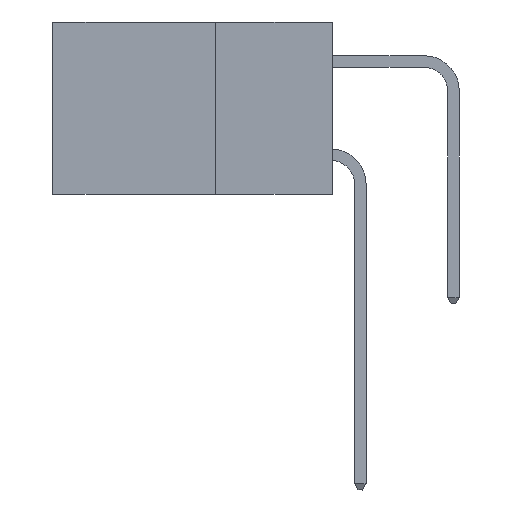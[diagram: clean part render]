
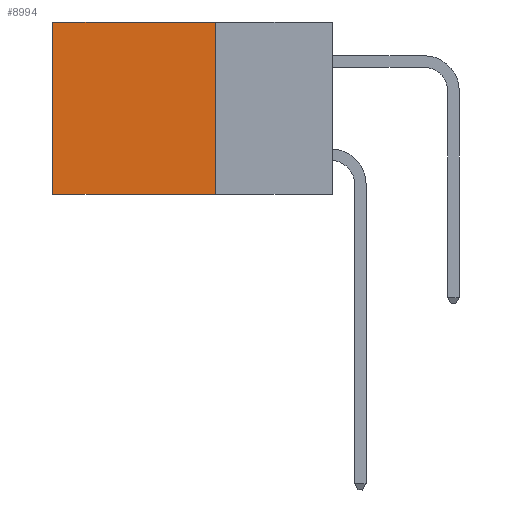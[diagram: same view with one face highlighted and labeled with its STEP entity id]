
A CAD part, left-side view. The second image highlights one B-rep face of the part: STEP entity #8994.
In plain terms, the highlighted planar face has unit normal (-1, 0, 0).
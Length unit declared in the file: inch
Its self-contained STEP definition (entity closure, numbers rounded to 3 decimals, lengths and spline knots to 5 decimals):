
#32 = PLANE ( 'NONE',  #10204 ) ;
#235 = LINE ( 'NONE', #8514, #19028 ) ;
#2487 = VECTOR ( 'NONE', #20587, 39.37008 ) ;
#2518 = LINE ( 'NONE', #22984, #2487 ) ;
#2733 = VERTEX_POINT ( 'NONE', #11501 ) ;
#2996 = CARTESIAN_POINT ( 'NONE',  ( 0.2615, 0.25, 0. ) ) ;
#5278 = EDGE_CURVE ( 'NONE', #16045, #2733, #235, .T. ) ;
#5744 = ORIENTED_EDGE ( 'NONE', *, *, #19781, .F. ) ;
#6216 = CARTESIAN_POINT ( 'NONE',  ( 0.2615, 0.25, -0.37 ) ) ;
#7022 = CARTESIAN_POINT ( 'NONE',  ( 0.2615, 0.25, 0. ) ) ;
#7184 = LINE ( 'NONE', #17378, #13124 ) ;
#7580 = DIRECTION ( 'NONE',  ( 0., 1., 0. ) ) ;
#8514 = CARTESIAN_POINT ( 'NONE',  ( 0.2615, 0.6, -0.37 ) ) ;
#8994 = ADVANCED_FACE ( 'NONE', ( #18244 ), #32, .F. ) ;
#9615 = VERTEX_POINT ( 'NONE', #6216 ) ;
#10204 = AXIS2_PLACEMENT_3D ( 'NONE', #24388, #17023, #25290 ) ;
#11501 = CARTESIAN_POINT ( 'NONE',  ( 0.2615, 0.6, -0.37 ) ) ;
#13116 = CARTESIAN_POINT ( 'NONE',  ( 0.2615, 0.6, 0. ) ) ;
#13124 = VECTOR ( 'NONE', #7580, 39.37008 ) ;
#13765 = EDGE_CURVE ( 'NONE', #16573, #16045, #14827, .T. ) ;
#14450 = ORIENTED_EDGE ( 'NONE', *, *, #13765, .T. ) ;
#14827 = LINE ( 'NONE', #7022, #17123 ) ;
#16045 = VERTEX_POINT ( 'NONE', #13116 ) ;
#16573 = VERTEX_POINT ( 'NONE', #2996 ) ;
#17023 = DIRECTION ( 'NONE',  ( 1., 0., 0. ) ) ;
#17123 = VECTOR ( 'NONE', #21084, 39.37008 ) ;
#17378 = CARTESIAN_POINT ( 'NONE',  ( 0.2615, 0.25, -0.37 ) ) ;
#18244 = FACE_OUTER_BOUND ( 'NONE', #24259, .T. ) ;
#19028 = VECTOR ( 'NONE', #22591, 39.37008 ) ;
#19781 = EDGE_CURVE ( 'NONE', #16573, #9615, #2518, .T. ) ;
#20270 = ORIENTED_EDGE ( 'NONE', *, *, #5278, .T. ) ;
#20587 = DIRECTION ( 'NONE',  ( 0., 0., -1. ) ) ;
#20787 = ORIENTED_EDGE ( 'NONE', *, *, #22605, .F. ) ;
#21084 = DIRECTION ( 'NONE',  ( 0., 1., 0. ) ) ;
#22591 = DIRECTION ( 'NONE',  ( 0., 0., -1. ) ) ;
#22605 = EDGE_CURVE ( 'NONE', #9615, #2733, #7184, .T. ) ;
#22984 = CARTESIAN_POINT ( 'NONE',  ( 0.2615, 0.25, -0.37 ) ) ;
#24259 = EDGE_LOOP ( 'NONE', ( #20270, #20787, #5744, #14450 ) ) ;
#24388 = CARTESIAN_POINT ( 'NONE',  ( 0.2615, 0.25, -0.37 ) ) ;
#25290 = DIRECTION ( 'NONE',  ( 0., 0., -1. ) ) ;
